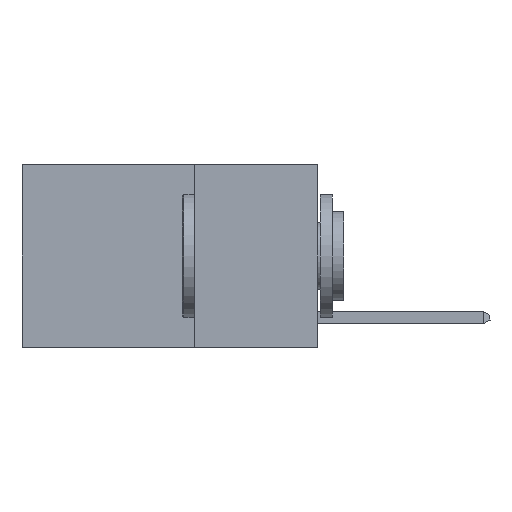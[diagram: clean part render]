
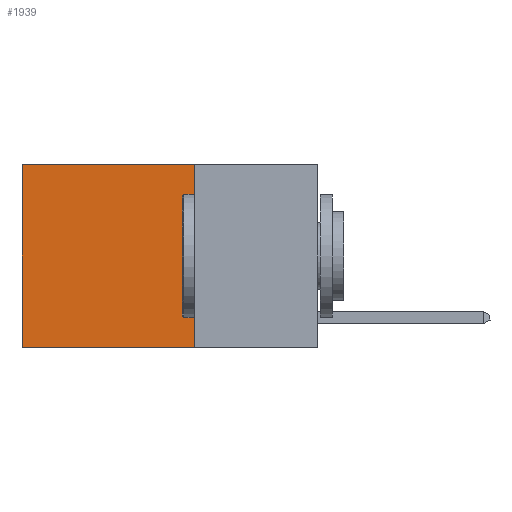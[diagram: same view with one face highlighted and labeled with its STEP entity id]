
A CAD part, left-side view. The second image highlights one B-rep face of the part: STEP entity #1939.
In plain terms, the highlighted planar face has unit normal (-1, 0, 0).
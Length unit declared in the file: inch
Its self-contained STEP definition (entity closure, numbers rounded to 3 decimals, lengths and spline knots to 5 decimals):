
#171 = VERTEX_POINT ( 'NONE', #18997 ) ;
#321 = AXIS2_PLACEMENT_3D ( 'NONE', #10555, #13606, #4643 ) ;
#550 = LINE ( 'NONE', #12882, #16047 ) ;
#889 = ORIENTED_EDGE ( 'NONE', *, *, #8309, .F. ) ;
#1424 = ORIENTED_EDGE ( 'NONE', *, *, #1472, .T. ) ;
#1472 = EDGE_CURVE ( 'NONE', #3377, #13825, #3931, .T. ) ;
#1681 = DIRECTION ( 'NONE',  ( 0., 1., 0. ) ) ;
#1939 = ADVANCED_FACE ( 'NONE', ( #4386 ), #12099, .F. ) ;
#2564 = EDGE_CURVE ( 'NONE', #171, #15653, #9058, .T. ) ;
#3377 = VERTEX_POINT ( 'NONE', #8021 ) ;
#3902 = DIRECTION ( 'NONE',  ( 0., 0., -1. ) ) ;
#3931 = LINE ( 'NONE', #11096, #7930 ) ;
#4386 = FACE_OUTER_BOUND ( 'NONE', #18454, .T. ) ;
#4643 = DIRECTION ( 'NONE',  ( 0., 0., -1. ) ) ;
#4713 = CARTESIAN_POINT ( 'NONE',  ( 0.2625, 0.6, 0. ) ) ;
#4829 = DIRECTION ( 'NONE',  ( 0., 0., -1. ) ) ;
#5073 = VECTOR ( 'NONE', #1681, 39.37008 ) ;
#5427 = EDGE_CURVE ( 'NONE', #13825, #15653, #6084, .T. ) ;
#6084 = LINE ( 'NONE', #15303, #9585 ) ;
#6161 = CARTESIAN_POINT ( 'NONE',  ( 0.2625, 0.25, -0.37 ) ) ;
#6433 = ORIENTED_EDGE ( 'NONE', *, *, #2564, .F. ) ;
#7930 = VECTOR ( 'NONE', #15534, 39.37008 ) ;
#8021 = CARTESIAN_POINT ( 'NONE',  ( 0.2625, 0.25, 0. ) ) ;
#8309 = EDGE_CURVE ( 'NONE', #3377, #171, #550, .T. ) ;
#9058 = LINE ( 'NONE', #6161, #5073 ) ;
#9585 = VECTOR ( 'NONE', #4829, 39.37008 ) ;
#10290 = CARTESIAN_POINT ( 'NONE',  ( 0.2625, 0.6, -0.37 ) ) ;
#10555 = CARTESIAN_POINT ( 'NONE',  ( 0.2625, 0.25, 0. ) ) ;
#11096 = CARTESIAN_POINT ( 'NONE',  ( 0.2625, 0.25, 0. ) ) ;
#12099 = PLANE ( 'NONE',  #321 ) ;
#12838 = ORIENTED_EDGE ( 'NONE', *, *, #5427, .T. ) ;
#12882 = CARTESIAN_POINT ( 'NONE',  ( 0.2625, 0.25, 0. ) ) ;
#13606 = DIRECTION ( 'NONE',  ( 1., 0., 0. ) ) ;
#13825 = VERTEX_POINT ( 'NONE', #4713 ) ;
#15303 = CARTESIAN_POINT ( 'NONE',  ( 0.2625, 0.6, 0. ) ) ;
#15534 = DIRECTION ( 'NONE',  ( 0., 1., 0. ) ) ;
#15653 = VERTEX_POINT ( 'NONE', #10290 ) ;
#16047 = VECTOR ( 'NONE', #3902, 39.37008 ) ;
#18454 = EDGE_LOOP ( 'NONE', ( #12838, #6433, #889, #1424 ) ) ;
#18997 = CARTESIAN_POINT ( 'NONE',  ( 0.2625, 0.25, -0.37 ) ) ;
